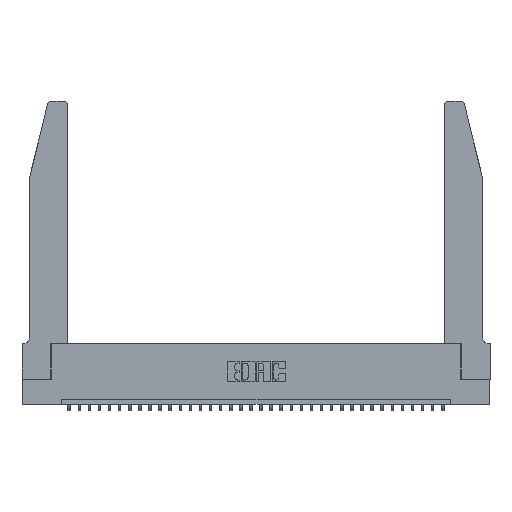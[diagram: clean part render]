
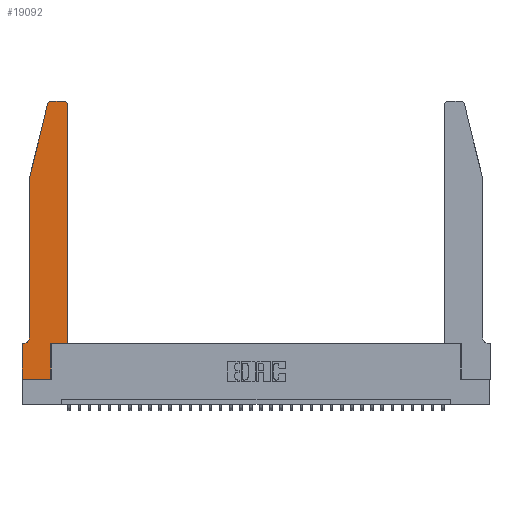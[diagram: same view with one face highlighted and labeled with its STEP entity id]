
A CAD part, top view. The second image highlights one B-rep face of the part: STEP entity #19092.
In plain terms, the highlighted planar face has unit normal (0, 0, 1).
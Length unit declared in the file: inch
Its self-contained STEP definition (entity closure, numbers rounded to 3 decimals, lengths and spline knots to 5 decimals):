
#129 = CARTESIAN_POINT ( 'NONE',  ( 0.0055, 0.35, 0.37 ) ) ;
#294 = ORIENTED_EDGE ( 'NONE', *, *, #21614, .T. ) ;
#410 = CARTESIAN_POINT ( 'NONE',  ( 0.2865, 0.35, 0.37 ) ) ;
#563 = VERTEX_POINT ( 'NONE', #29023 ) ;
#751 = CARTESIAN_POINT ( 'NONE',  ( 0.2865, 0., 0.37 ) ) ;
#817 = DIRECTION ( 'NONE',  ( 0., 1., 0. ) ) ;
#1207 = EDGE_CURVE ( 'NONE', #7374, #21493, #9985, .T. ) ;
#1754 = DIRECTION ( 'NONE',  ( -1., 0., 0. ) ) ;
#1930 = CARTESIAN_POINT ( 'NONE',  ( 0.0755, 2., 0.37 ) ) ;
#2412 = ORIENTED_EDGE ( 'NONE', *, *, #30042, .T. ) ;
#3398 = EDGE_CURVE ( 'NONE', #7940, #24781, #33562, .T. ) ;
#3582 = CARTESIAN_POINT ( 'NONE',  ( 0.4505, 0.35, 0.37 ) ) ;
#3748 = CIRCLE ( 'NONE', #15294, 0.07 ) ;
#4338 = VECTOR ( 'NONE', #7246, 39.37008 ) ;
#4473 = DIRECTION ( 'NONE',  ( 0., 0., 1. ) ) ;
#4744 = ORIENTED_EDGE ( 'NONE', *, *, #7089, .T. ) ;
#5109 = DIRECTION ( 'NONE',  ( 0., 0., -1. ) ) ;
#5654 = VERTEX_POINT ( 'NONE', #6722 ) ;
#6080 = EDGE_CURVE ( 'NONE', #7105, #26642, #12577, .T. ) ;
#6124 = DIRECTION ( 'NONE',  ( 0., 0., 1. ) ) ;
#6261 = CIRCLE ( 'NONE', #9301, 0.03 ) ;
#6335 = VECTOR ( 'NONE', #817, 39.37008 ) ;
#6722 = CARTESIAN_POINT ( 'NONE',  ( 0.4505, 0.35, 0.37 ) ) ;
#7089 = EDGE_CURVE ( 'NONE', #5654, #7374, #20263, .T. ) ;
#7105 = VERTEX_POINT ( 'NONE', #16130 ) ;
#7214 = ORIENTED_EDGE ( 'NONE', *, *, #9751, .T. ) ;
#7246 = DIRECTION ( 'NONE',  ( 0., -1., 0. ) ) ;
#7374 = VERTEX_POINT ( 'NONE', #30282 ) ;
#7940 = VERTEX_POINT ( 'NONE', #751 ) ;
#8276 = ORIENTED_EDGE ( 'NONE', *, *, #27713, .T. ) ;
#8514 = VECTOR ( 'NONE', #11834, 39.37008 ) ;
#8559 = LINE ( 'NONE', #18844, #20885 ) ;
#8852 = CARTESIAN_POINT ( 'NONE',  ( 0.25487, 2.72718, 0.37 ) ) ;
#9076 = CARTESIAN_POINT ( 'NONE',  ( 0.4505, 0.35, 0.37 ) ) ;
#9250 = DIRECTION ( 'NONE',  ( 0., -1., 0. ) ) ;
#9252 = CARTESIAN_POINT ( 'NONE',  ( 0.2605, 2.75, 0.37 ) ) ;
#9301 = AXIS2_PLACEMENT_3D ( 'NONE', #21805, #6124, #24428 ) ;
#9497 = VERTEX_POINT ( 'NONE', #8852 ) ;
#9751 = EDGE_CURVE ( 'NONE', #21493, #9924, #25042, .T. ) ;
#9924 = VERTEX_POINT ( 'NONE', #26176 ) ;
#9985 = CIRCLE ( 'NONE', #32718, 0.03 ) ;
#10938 = LINE ( 'NONE', #33184, #14252 ) ;
#10956 = CARTESIAN_POINT ( 'NONE',  ( 0.0755, 0.42, 0.37 ) ) ;
#11433 = EDGE_CURVE ( 'NONE', #19835, #22117, #31849, .T. ) ;
#11834 = DIRECTION ( 'NONE',  ( 0., 1., 0. ) ) ;
#12468 = CARTESIAN_POINT ( 'NONE',  ( 0.0755, 0.35, 0.37 ) ) ;
#12577 = LINE ( 'NONE', #1930, #4338 ) ;
#12746 = CARTESIAN_POINT ( 'NONE',  ( 0., 0., 0.37 ) ) ;
#13059 = VECTOR ( 'NONE', #28096, 39.37008 ) ;
#14252 = VECTOR ( 'NONE', #9250, 39.37008 ) ;
#15294 = AXIS2_PLACEMENT_3D ( 'NONE', #20812, #5109, #26049 ) ;
#15396 = DIRECTION ( 'NONE',  ( 1., 0., 0. ) ) ;
#16101 = ORIENTED_EDGE ( 'NONE', *, *, #3398, .T. ) ;
#16130 = CARTESIAN_POINT ( 'NONE',  ( 0.0755, 2., 0.37 ) ) ;
#16392 = DIRECTION ( 'NONE',  ( -0.239, -0.971, 0. ) ) ;
#16405 = EDGE_CURVE ( 'NONE', #9497, #7105, #8559, .T. ) ;
#17116 = LINE ( 'NONE', #12746, #26498 ) ;
#17650 = PLANE ( 'NONE',  #20939 ) ;
#17763 = ORIENTED_EDGE ( 'NONE', *, *, #22019, .T. ) ;
#17769 = ORIENTED_EDGE ( 'NONE', *, *, #16405, .T. ) ;
#18844 = CARTESIAN_POINT ( 'NONE',  ( 0.0755, 2., 0.37 ) ) ;
#19092 = ADVANCED_FACE ( 'NONE', ( #33442 ), #17650, .T. ) ;
#19273 = VECTOR ( 'NONE', #27709, 39.37008 ) ;
#19835 = VERTEX_POINT ( 'NONE', #129 ) ;
#19988 = DIRECTION ( 'NONE',  ( 1., 0., 0. ) ) ;
#20155 = CARTESIAN_POINT ( 'NONE',  ( 0., 0.35, 0.37 ) ) ;
#20263 = LINE ( 'NONE', #3582, #6335 ) ;
#20812 = CARTESIAN_POINT ( 'NONE',  ( 0.0055, 0.42, 0.37 ) ) ;
#20885 = VECTOR ( 'NONE', #16392, 39.37008 ) ;
#20939 = AXIS2_PLACEMENT_3D ( 'NONE', #20155, #4473, #15396 ) ;
#21493 = VERTEX_POINT ( 'NONE', #23327 ) ;
#21614 = EDGE_CURVE ( 'NONE', #26642, #19835, #3748, .T. ) ;
#21654 = ORIENTED_EDGE ( 'NONE', *, *, #28183, .T. ) ;
#21805 = CARTESIAN_POINT ( 'NONE',  ( 0.284, 2.72, 0.37 ) ) ;
#22019 = EDGE_CURVE ( 'NONE', #24781, #5654, #23463, .T. ) ;
#22117 = VERTEX_POINT ( 'NONE', #25331 ) ;
#22301 = DIRECTION ( 'NONE',  ( 0., 0., 1. ) ) ;
#23327 = CARTESIAN_POINT ( 'NONE',  ( 0.4205, 2.75, 0.37 ) ) ;
#23463 = LINE ( 'NONE', #9076, #19273 ) ;
#24428 = DIRECTION ( 'NONE',  ( 1., 0., 0. ) ) ;
#24781 = VERTEX_POINT ( 'NONE', #410 ) ;
#25042 = LINE ( 'NONE', #9252, #30756 ) ;
#25189 = ORIENTED_EDGE ( 'NONE', *, *, #6080, .T. ) ;
#25331 = CARTESIAN_POINT ( 'NONE',  ( 0., 0.35, 0.37 ) ) ;
#26049 = DIRECTION ( 'NONE',  ( -1., 0., 0. ) ) ;
#26176 = CARTESIAN_POINT ( 'NONE',  ( 0.284, 2.75, 0.37 ) ) ;
#26498 = VECTOR ( 'NONE', #31029, 39.37008 ) ;
#26642 = VERTEX_POINT ( 'NONE', #10956 ) ;
#27709 = DIRECTION ( 'NONE',  ( 1., 0., 0. ) ) ;
#27713 = EDGE_CURVE ( 'NONE', #563, #7940, #17116, .T. ) ;
#28096 = DIRECTION ( 'NONE',  ( -1., 0., 0. ) ) ;
#28183 = EDGE_CURVE ( 'NONE', #22117, #563, #10938, .T. ) ;
#29023 = CARTESIAN_POINT ( 'NONE',  ( 0., 0., 0.37 ) ) ;
#30000 = CARTESIAN_POINT ( 'NONE',  ( 0.2865, 0.35, 0.37 ) ) ;
#30042 = EDGE_CURVE ( 'NONE', #9924, #9497, #6261, .T. ) ;
#30282 = CARTESIAN_POINT ( 'NONE',  ( 0.4505, 2.72, 0.37 ) ) ;
#30756 = VECTOR ( 'NONE', #1754, 39.37008 ) ;
#31029 = DIRECTION ( 'NONE',  ( 1., 0., 0. ) ) ;
#31104 = ORIENTED_EDGE ( 'NONE', *, *, #1207, .T. ) ;
#31849 = LINE ( 'NONE', #12468, #13059 ) ;
#32284 = EDGE_LOOP ( 'NONE', ( #7214, #2412, #17769, #25189, #294, #33391, #21654, #8276, #16101, #17763, #4744, #31104 ) ) ;
#32718 = AXIS2_PLACEMENT_3D ( 'NONE', #33073, #22301, #19988 ) ;
#33073 = CARTESIAN_POINT ( 'NONE',  ( 0.4205, 2.72, 0.37 ) ) ;
#33184 = CARTESIAN_POINT ( 'NONE',  ( 0., 0., 0.37 ) ) ;
#33391 = ORIENTED_EDGE ( 'NONE', *, *, #11433, .T. ) ;
#33442 = FACE_OUTER_BOUND ( 'NONE', #32284, .T. ) ;
#33562 = LINE ( 'NONE', #30000, #8514 ) ;
